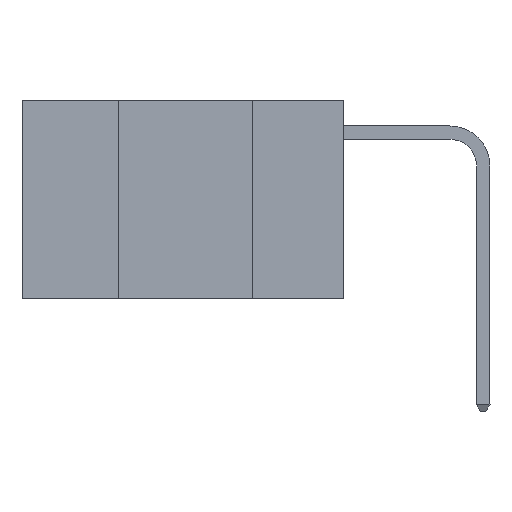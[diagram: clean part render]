
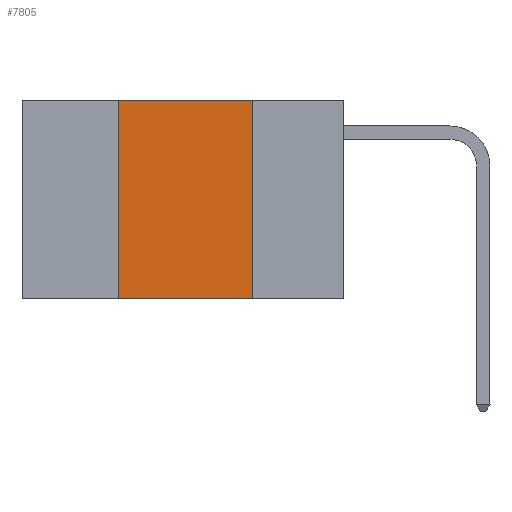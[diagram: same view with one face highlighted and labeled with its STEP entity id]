
A CAD part, left-side view. The second image highlights one B-rep face of the part: STEP entity #7805.
In plain terms, the highlighted planar face has unit normal (-1, 0, 0).
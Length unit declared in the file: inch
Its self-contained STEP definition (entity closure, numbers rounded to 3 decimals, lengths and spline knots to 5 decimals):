
#347 = AXIS2_PLACEMENT_3D ( 'NONE', #2895, #2051, #2012 ) ;
#1052 = VECTOR ( 'NONE', #4234, 39.37008 ) ;
#1079 = LINE ( 'NONE', #4189, #1052 ) ;
#1160 = VECTOR ( 'NONE', #5568, 39.37008 ) ;
#1990 = EDGE_CURVE ( 'NONE', #6869, #11336, #10869, .T. ) ;
#2012 = DIRECTION ( 'NONE',  ( 0., 0., -1. ) ) ;
#2051 = DIRECTION ( 'NONE',  ( 1., 0., 0. ) ) ;
#2472 = PLANE ( 'NONE',  #347 ) ;
#2590 = LINE ( 'NONE', #5611, #1160 ) ;
#2726 = EDGE_CURVE ( 'NONE', #6869, #11996, #2590, .T. ) ;
#2895 = CARTESIAN_POINT ( 'NONE',  ( 0., 0.6, 0. ) ) ;
#3060 = VERTEX_POINT ( 'NONE', #3536 ) ;
#3369 = CARTESIAN_POINT ( 'NONE',  ( 0., 0.17, -0.37 ) ) ;
#3536 = CARTESIAN_POINT ( 'NONE',  ( 0., 0.17, 0. ) ) ;
#4067 = FACE_OUTER_BOUND ( 'NONE', #10463, .T. ) ;
#4121 = EDGE_CURVE ( 'NONE', #3060, #11336, #1079, .T. ) ;
#4189 = CARTESIAN_POINT ( 'NONE',  ( 0., 0.17, 0. ) ) ;
#4234 = DIRECTION ( 'NONE',  ( 0., 0., -1. ) ) ;
#4839 = VECTOR ( 'NONE', #10374, 39.37008 ) ;
#5568 = DIRECTION ( 'NONE',  ( 0., 0., 1. ) ) ;
#5611 = CARTESIAN_POINT ( 'NONE',  ( 0., 0.42, 0. ) ) ;
#6869 = VERTEX_POINT ( 'NONE', #9148 ) ;
#7334 = ORIENTED_EDGE ( 'NONE', *, *, #4121, .F. ) ;
#7359 = ORIENTED_EDGE ( 'NONE', *, *, #8736, .F. ) ;
#7466 = ORIENTED_EDGE ( 'NONE', *, *, #2726, .F. ) ;
#7512 = ORIENTED_EDGE ( 'NONE', *, *, #1990, .T. ) ;
#7805 = ADVANCED_FACE ( 'NONE', ( #4067 ), #2472, .F. ) ;
#8736 = EDGE_CURVE ( 'NONE', #11996, #3060, #11830, .T. ) ;
#9148 = CARTESIAN_POINT ( 'NONE',  ( 0., 0.42, -0.37 ) ) ;
#10374 = DIRECTION ( 'NONE',  ( 0., -1., 0. ) ) ;
#10460 = CARTESIAN_POINT ( 'NONE',  ( 0., 0.6, 0. ) ) ;
#10463 = EDGE_LOOP ( 'NONE', ( #7334, #7359, #7466, #7512 ) ) ;
#10771 = VECTOR ( 'NONE', #10808, 39.37008 ) ;
#10808 = DIRECTION ( 'NONE',  ( 0., -1., 0. ) ) ;
#10869 = LINE ( 'NONE', #10999, #10771 ) ;
#10999 = CARTESIAN_POINT ( 'NONE',  ( 0., 0.6, -0.37 ) ) ;
#11336 = VERTEX_POINT ( 'NONE', #3369 ) ;
#11547 = CARTESIAN_POINT ( 'NONE',  ( 0., 0.42, 0. ) ) ;
#11830 = LINE ( 'NONE', #10460, #4839 ) ;
#11996 = VERTEX_POINT ( 'NONE', #11547 ) ;
